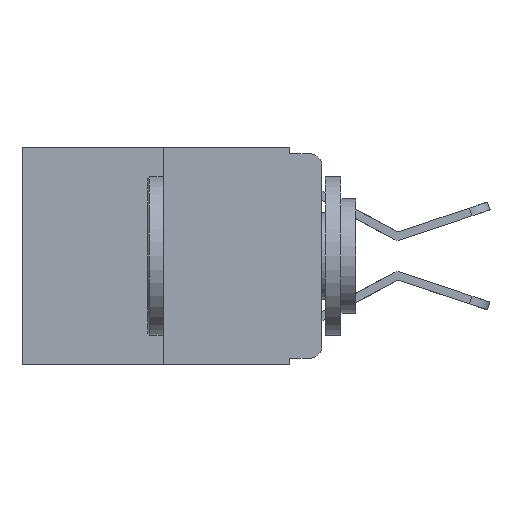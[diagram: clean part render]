
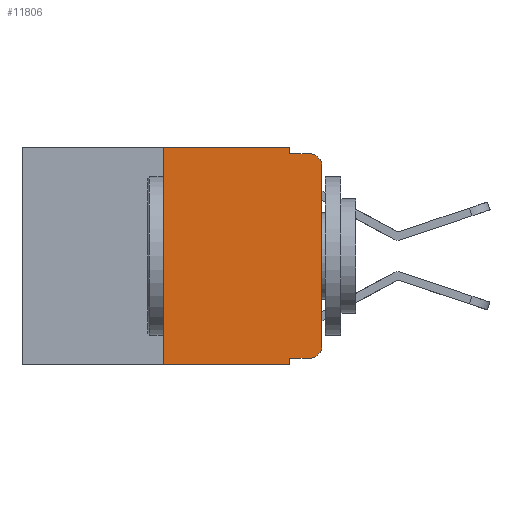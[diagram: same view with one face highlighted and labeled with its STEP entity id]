
A CAD part, left-side view. The second image highlights one B-rep face of the part: STEP entity #11806.
In plain terms, the highlighted planar face has unit normal (-1, 0, 0).
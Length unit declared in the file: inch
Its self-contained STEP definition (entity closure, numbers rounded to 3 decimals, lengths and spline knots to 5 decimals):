
#437 = VERTEX_POINT ( 'NONE', #817 ) ;
#556 = VECTOR ( 'NONE', #12434, 39.37008 ) ;
#661 = CARTESIAN_POINT ( 'NONE',  ( 0., 0.02, -0.333 ) ) ;
#817 = CARTESIAN_POINT ( 'NONE',  ( 0., 0.02, -0.01 ) ) ;
#839 = AXIS2_PLACEMENT_3D ( 'NONE', #5955, #13574, #2196 ) ;
#942 = VERTEX_POINT ( 'NONE', #12915 ) ;
#1348 = VECTOR ( 'NONE', #9562, 39.37008 ) ;
#1364 = EDGE_LOOP ( 'NONE', ( #8172, #8997, #2646, #2952, #11067, #23509, #5084, #12239, #2975, #11958 ) ) ;
#1379 = CARTESIAN_POINT ( 'NONE',  ( 0., 0.051, -0.01 ) ) ;
#1799 = EDGE_CURVE ( 'NONE', #942, #16206, #10715, .T. ) ;
#1894 = EDGE_CURVE ( 'NONE', #21875, #14779, #23103, .T. ) ;
#2196 = DIRECTION ( 'NONE',  ( 0., 0., -1. ) ) ;
#2646 = ORIENTED_EDGE ( 'NONE', *, *, #15763, .F. ) ;
#2952 = ORIENTED_EDGE ( 'NONE', *, *, #1894, .F. ) ;
#2975 = ORIENTED_EDGE ( 'NONE', *, *, #22679, .T. ) ;
#3212 = DIRECTION ( 'NONE',  ( 0., -1., 0. ) ) ;
#3213 = VECTOR ( 'NONE', #7163, 39.37008 ) ;
#3252 = CARTESIAN_POINT ( 'NONE',  ( 0., 0.25, 0. ) ) ;
#3394 = CARTESIAN_POINT ( 'NONE',  ( 0., 0.02, -0.03 ) ) ;
#3937 = EDGE_CURVE ( 'NONE', #18755, #437, #12931, .T. ) ;
#5084 = ORIENTED_EDGE ( 'NONE', *, *, #1799, .T. ) ;
#5338 = DIRECTION ( 'NONE',  ( 0., 0., -1. ) ) ;
#5888 = DIRECTION ( 'NONE',  ( -1., 0., 0. ) ) ;
#5955 = CARTESIAN_POINT ( 'NONE',  ( 0., 0.473, 0. ) ) ;
#6029 = AXIS2_PLACEMENT_3D ( 'NONE', #17094, #5888, #18918 ) ;
#6186 = LINE ( 'NONE', #12818, #20400 ) ;
#7080 = CARTESIAN_POINT ( 'NONE',  ( 0., 0.051, 0. ) ) ;
#7163 = DIRECTION ( 'NONE',  ( 0., 0., -1. ) ) ;
#7650 = CARTESIAN_POINT ( 'NONE',  ( 0., 0., 0. ) ) ;
#7699 = DIRECTION ( 'NONE',  ( 0., 0., 1. ) ) ;
#8172 = ORIENTED_EDGE ( 'NONE', *, *, #17734, .T. ) ;
#8535 = VECTOR ( 'NONE', #7699, 39.37008 ) ;
#8601 = AXIS2_PLACEMENT_3D ( 'NONE', #3394, #16569, #5338 ) ;
#8691 = VERTEX_POINT ( 'NONE', #661 ) ;
#8765 = EDGE_CURVE ( 'NONE', #14809, #16206, #14902, .T. ) ;
#8997 = ORIENTED_EDGE ( 'NONE', *, *, #3937, .T. ) ;
#9562 = DIRECTION ( 'NONE',  ( 0., 0., 1. ) ) ;
#10346 = VERTEX_POINT ( 'NONE', #3252 ) ;
#10449 = CARTESIAN_POINT ( 'NONE',  ( 0., 0.051, 0. ) ) ;
#10715 = LINE ( 'NONE', #14996, #556 ) ;
#11067 = ORIENTED_EDGE ( 'NONE', *, *, #15185, .F. ) ;
#11806 = ADVANCED_FACE ( 'NONE', ( #18151 ), #22553, .F. ) ;
#11958 = ORIENTED_EDGE ( 'NONE', *, *, #19110, .T. ) ;
#12239 = ORIENTED_EDGE ( 'NONE', *, *, #8765, .F. ) ;
#12434 = DIRECTION ( 'NONE',  ( 0., -1., 0. ) ) ;
#12818 = CARTESIAN_POINT ( 'NONE',  ( 0., 0.051, -0.01 ) ) ;
#12915 = CARTESIAN_POINT ( 'NONE',  ( 0., 0.25, -0.343 ) ) ;
#12931 = CIRCLE ( 'NONE', #8601, 0.02 ) ;
#13537 = LINE ( 'NONE', #20557, #8535 ) ;
#13574 = DIRECTION ( 'NONE',  ( 1., 0., 0. ) ) ;
#14070 = LINE ( 'NONE', #14473, #14656 ) ;
#14473 = CARTESIAN_POINT ( 'NONE',  ( 0., 0.051, -0.333 ) ) ;
#14656 = VECTOR ( 'NONE', #3212, 39.37008 ) ;
#14779 = VERTEX_POINT ( 'NONE', #1379 ) ;
#14809 = VERTEX_POINT ( 'NONE', #21837 ) ;
#14902 = LINE ( 'NONE', #21346, #23861 ) ;
#14996 = CARTESIAN_POINT ( 'NONE',  ( 0., 0.473, -0.343 ) ) ;
#15185 = EDGE_CURVE ( 'NONE', #10346, #21875, #23199, .T. ) ;
#15650 = CIRCLE ( 'NONE', #6029, 0.02 ) ;
#15763 = EDGE_CURVE ( 'NONE', #14779, #437, #6186, .T. ) ;
#15780 = LINE ( 'NONE', #7650, #1348 ) ;
#15910 = DIRECTION ( 'NONE',  ( 0., 0., -1. ) ) ;
#16072 = CARTESIAN_POINT ( 'NONE',  ( 0., 0., -0.03 ) ) ;
#16206 = VERTEX_POINT ( 'NONE', #23111 ) ;
#16569 = DIRECTION ( 'NONE',  ( -1., 0., 0. ) ) ;
#17094 = CARTESIAN_POINT ( 'NONE',  ( 0., 0.02, -0.313 ) ) ;
#17734 = EDGE_CURVE ( 'NONE', #18555, #18755, #15780, .T. ) ;
#18151 = FACE_OUTER_BOUND ( 'NONE', #1364, .T. ) ;
#18423 = CARTESIAN_POINT ( 'NONE',  ( 0., 0.473, 0. ) ) ;
#18555 = VERTEX_POINT ( 'NONE', #19091 ) ;
#18755 = VERTEX_POINT ( 'NONE', #16072 ) ;
#18918 = DIRECTION ( 'NONE',  ( 0., 0., -1. ) ) ;
#19035 = VECTOR ( 'NONE', #20224, 39.37008 ) ;
#19091 = CARTESIAN_POINT ( 'NONE',  ( 0., 0., -0.313 ) ) ;
#19110 = EDGE_CURVE ( 'NONE', #8691, #18555, #15650, .T. ) ;
#20224 = DIRECTION ( 'NONE',  ( 0., -1., 0. ) ) ;
#20400 = VECTOR ( 'NONE', #23668, 39.37008 ) ;
#20557 = CARTESIAN_POINT ( 'NONE',  ( 0., 0.25, 0. ) ) ;
#21346 = CARTESIAN_POINT ( 'NONE',  ( 0., 0.051, 0. ) ) ;
#21837 = CARTESIAN_POINT ( 'NONE',  ( 0., 0.051, -0.333 ) ) ;
#21875 = VERTEX_POINT ( 'NONE', #10449 ) ;
#22237 = EDGE_CURVE ( 'NONE', #942, #10346, #13537, .T. ) ;
#22553 = PLANE ( 'NONE',  #839 ) ;
#22679 = EDGE_CURVE ( 'NONE', #14809, #8691, #14070, .T. ) ;
#23103 = LINE ( 'NONE', #7080, #3213 ) ;
#23111 = CARTESIAN_POINT ( 'NONE',  ( 0., 0.051, -0.343 ) ) ;
#23199 = LINE ( 'NONE', #18423, #19035 ) ;
#23509 = ORIENTED_EDGE ( 'NONE', *, *, #22237, .F. ) ;
#23668 = DIRECTION ( 'NONE',  ( 0., -1., 0. ) ) ;
#23861 = VECTOR ( 'NONE', #15910, 39.37008 ) ;
